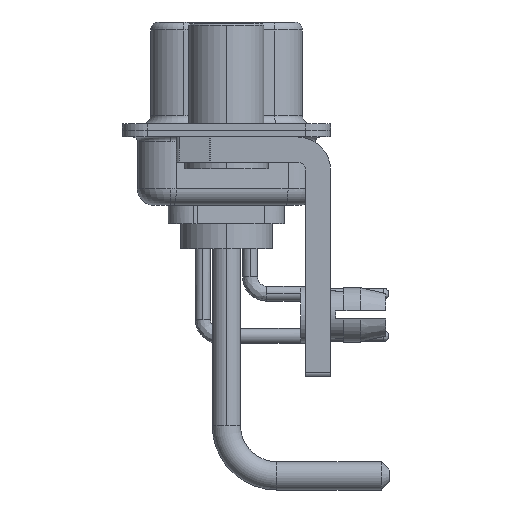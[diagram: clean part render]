
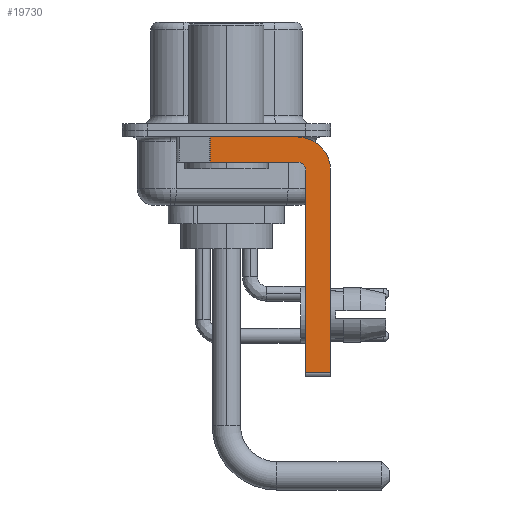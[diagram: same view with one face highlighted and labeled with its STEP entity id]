
A CAD part, left-side view. The second image highlights one B-rep face of the part: STEP entity #19730.
In plain terms, the highlighted planar face has unit normal (-1, 0, 0).
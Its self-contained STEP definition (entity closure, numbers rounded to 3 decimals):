
#345 = DIRECTION ( 'NONE',  ( 0., 0., -1. ) ) ;
#1654 = VECTOR ( 'NONE', #3977, 1000. ) ;
#2258 = DIRECTION ( 'NONE',  ( 1., 0., 0. ) ) ;
#2295 = DIRECTION ( 'NONE',  ( 0., 0., -1. ) ) ;
#2356 = CARTESIAN_POINT ( 'NONE',  ( -2.9, -4.25, -2.4 ) ) ;
#2878 = VECTOR ( 'NONE', #5826, 1000. ) ;
#2927 = EDGE_CURVE ( 'NONE', #22617, #19344, #24530, .T. ) ;
#3788 = CARTESIAN_POINT ( 'NONE',  ( -2.9, -4.75, -2.4 ) ) ;
#3941 = DIRECTION ( 'NONE',  ( 0., 1., 0. ) ) ;
#3977 = DIRECTION ( 'NONE',  ( 0., 0., 1. ) ) ;
#4232 = CARTESIAN_POINT ( 'NONE',  ( -2.9, 0.978, -0.4 ) ) ;
#4435 = LINE ( 'NONE', #20723, #25844 ) ;
#4490 = AXIS2_PLACEMENT_3D ( 'NONE', #2356, #25194, #6255 ) ;
#4816 = EDGE_CURVE ( 'NONE', #12962, #21435, #25207, .T. ) ;
#5819 = EDGE_LOOP ( 'NONE', ( #16252, #24294, #21903, #13753, #11123, #22027, #19731, #11723 ) ) ;
#5826 = DIRECTION ( 'NONE',  ( 0., -1., 0. ) ) ;
#6255 = DIRECTION ( 'NONE',  ( 0., 0., 1. ) ) ;
#6367 = CARTESIAN_POINT ( 'NONE',  ( -2.9, -4.25, -1.9 ) ) ;
#6800 = LINE ( 'NONE', #21328, #16112 ) ;
#8299 = PLANE ( 'NONE',  #25448 ) ;
#8504 = LINE ( 'NONE', #16711, #2878 ) ;
#9691 = DIRECTION ( 'NONE',  ( 0., 0., -1. ) ) ;
#9892 = EDGE_CURVE ( 'NONE', #15881, #18528, #8504, .T. ) ;
#10082 = EDGE_CURVE ( 'NONE', #18528, #12962, #19232, .T. ) ;
#10317 = CARTESIAN_POINT ( 'NONE',  ( -2.9, -4.25, -2.4 ) ) ;
#10414 = CARTESIAN_POINT ( 'NONE',  ( -2.9, -4.25, -1.9 ) ) ;
#10465 = DIRECTION ( 'NONE',  ( 0., 0., -1. ) ) ;
#10910 = CIRCLE ( 'NONE', #4490, 0.5 ) ;
#11123 = ORIENTED_EDGE ( 'NONE', *, *, #11306, .F. ) ;
#11306 = EDGE_CURVE ( 'NONE', #24272, #13244, #22278, .T. ) ;
#11723 = ORIENTED_EDGE ( 'NONE', *, *, #10082, .F. ) ;
#12304 = CARTESIAN_POINT ( 'NONE',  ( -2.9, -6.25, -14.55 ) ) ;
#12312 = CARTESIAN_POINT ( 'NONE',  ( -2.9, -4.75, -14.8 ) ) ;
#12354 = AXIS2_PLACEMENT_3D ( 'NONE', #23946, #19923, #9691 ) ;
#12962 = VERTEX_POINT ( 'NONE', #24688 ) ;
#13244 = VERTEX_POINT ( 'NONE', #3788 ) ;
#13753 = ORIENTED_EDGE ( 'NONE', *, *, #25308, .F. ) ;
#14277 = CARTESIAN_POINT ( 'NONE',  ( -2.9, -4.25, -0.4 ) ) ;
#14982 = CARTESIAN_POINT ( 'NONE',  ( -2.9, -6.25, -2.4 ) ) ;
#15744 = CARTESIAN_POINT ( 'NONE',  ( -2.9, -4.75, -14.55 ) ) ;
#15881 = VERTEX_POINT ( 'NONE', #4232 ) ;
#16112 = VECTOR ( 'NONE', #16887, 1000. ) ;
#16252 = ORIENTED_EDGE ( 'NONE', *, *, #9892, .F. ) ;
#16711 = CARTESIAN_POINT ( 'NONE',  ( -2.9, 3., -0.4 ) ) ;
#16887 = DIRECTION ( 'NONE',  ( 0., -1., 0. ) ) ;
#17511 = VECTOR ( 'NONE', #345, 1000. ) ;
#18528 = VERTEX_POINT ( 'NONE', #14277 ) ;
#19232 = CIRCLE ( 'NONE', #12354, 2. ) ;
#19344 = VERTEX_POINT ( 'NONE', #24613 ) ;
#19730 = ADVANCED_FACE ( 'NONE', ( #24580 ), #8299, .F. ) ;
#19731 = ORIENTED_EDGE ( 'NONE', *, *, #4816, .F. ) ;
#19923 = DIRECTION ( 'NONE',  ( 1., 0., 0. ) ) ;
#20651 = EDGE_CURVE ( 'NONE', #15881, #19344, #4435, .T. ) ;
#20723 = CARTESIAN_POINT ( 'NONE',  ( -2.9, 0.978, -1.9 ) ) ;
#21328 = CARTESIAN_POINT ( 'NONE',  ( -2.9, -4.25, -14.55 ) ) ;
#21435 = VERTEX_POINT ( 'NONE', #12304 ) ;
#21903 = ORIENTED_EDGE ( 'NONE', *, *, #2927, .F. ) ;
#22027 = ORIENTED_EDGE ( 'NONE', *, *, #26289, .T. ) ;
#22029 = VECTOR ( 'NONE', #3941, 1000. ) ;
#22278 = LINE ( 'NONE', #12312, #1654 ) ;
#22617 = VERTEX_POINT ( 'NONE', #10414 ) ;
#23946 = CARTESIAN_POINT ( 'NONE',  ( -2.9, -4.25, -2.4 ) ) ;
#24272 = VERTEX_POINT ( 'NONE', #15744 ) ;
#24294 = ORIENTED_EDGE ( 'NONE', *, *, #20651, .T. ) ;
#24530 = LINE ( 'NONE', #6367, #22029 ) ;
#24580 = FACE_OUTER_BOUND ( 'NONE', #5819, .T. ) ;
#24613 = CARTESIAN_POINT ( 'NONE',  ( -2.9, 0.978, -1.9 ) ) ;
#24688 = CARTESIAN_POINT ( 'NONE',  ( -2.9, -6.25, -2.4 ) ) ;
#25194 = DIRECTION ( 'NONE',  ( -1., 0., 0. ) ) ;
#25207 = LINE ( 'NONE', #14982, #17511 ) ;
#25308 = EDGE_CURVE ( 'NONE', #13244, #22617, #10910, .T. ) ;
#25448 = AXIS2_PLACEMENT_3D ( 'NONE', #10317, #2258, #10465 ) ;
#25844 = VECTOR ( 'NONE', #2295, 1000. ) ;
#26289 = EDGE_CURVE ( 'NONE', #24272, #21435, #6800, .T. ) ;
